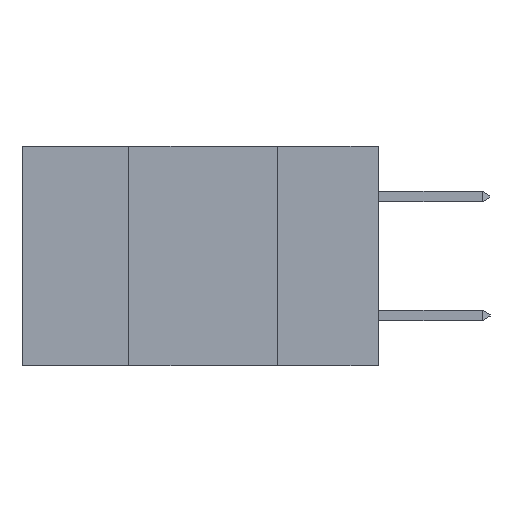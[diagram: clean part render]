
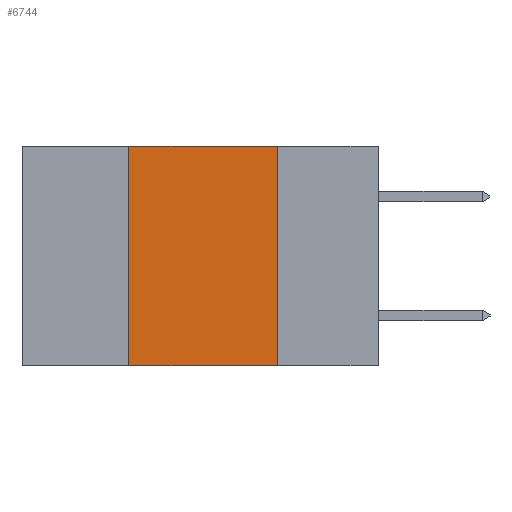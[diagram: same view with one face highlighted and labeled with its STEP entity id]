
A CAD part, left-side view. The second image highlights one B-rep face of the part: STEP entity #6744.
In plain terms, the highlighted planar face has unit normal (-1, 0, 0).
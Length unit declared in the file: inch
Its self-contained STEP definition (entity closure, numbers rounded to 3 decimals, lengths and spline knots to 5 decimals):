
#1080 = EDGE_LOOP ( 'NONE', ( #16471, #5968, #16943, #7786 ) ) ;
#1259 = VERTEX_POINT ( 'NONE', #9076 ) ;
#2033 = VECTOR ( 'NONE', #11052, 39.37008 ) ;
#2097 = VERTEX_POINT ( 'NONE', #18645 ) ;
#4067 = VERTEX_POINT ( 'NONE', #17515 ) ;
#4369 = CARTESIAN_POINT ( 'NONE',  ( 0., 0.6, -0.37 ) ) ;
#4642 = PLANE ( 'NONE',  #17692 ) ;
#4816 = CARTESIAN_POINT ( 'NONE',  ( 0., 0.42, 0. ) ) ;
#5235 = VECTOR ( 'NONE', #6069, 39.37008 ) ;
#5297 = FACE_OUTER_BOUND ( 'NONE', #1080, .T. ) ;
#5775 = LINE ( 'NONE', #4369, #5235 ) ;
#5968 = ORIENTED_EDGE ( 'NONE', *, *, #6484, .F. ) ;
#6069 = DIRECTION ( 'NONE',  ( 0., -1., 0. ) ) ;
#6484 = EDGE_CURVE ( 'NONE', #22376, #2097, #22396, .T. ) ;
#6744 = ADVANCED_FACE ( 'NONE', ( #5297 ), #4642, .F. ) ;
#7272 = CARTESIAN_POINT ( 'NONE',  ( 0., 0.42, -0.37 ) ) ;
#7786 = ORIENTED_EDGE ( 'NONE', *, *, #8800, .T. ) ;
#8374 = EDGE_CURVE ( 'NONE', #1259, #22376, #18796, .T. ) ;
#8800 = EDGE_CURVE ( 'NONE', #1259, #4067, #5775, .T. ) ;
#9076 = CARTESIAN_POINT ( 'NONE',  ( 0., 0.42, -0.37 ) ) ;
#9968 = DIRECTION ( 'NONE',  ( 1., 0., 0. ) ) ;
#10836 = DIRECTION ( 'NONE',  ( 0., 0., 1. ) ) ;
#11052 = DIRECTION ( 'NONE',  ( 0., -1., 0. ) ) ;
#12352 = LINE ( 'NONE', #13141, #21150 ) ;
#13141 = CARTESIAN_POINT ( 'NONE',  ( 0., 0.17, -0.37 ) ) ;
#13564 = EDGE_CURVE ( 'NONE', #2097, #4067, #12352, .T. ) ;
#14099 = VECTOR ( 'NONE', #10836, 39.37008 ) ;
#14932 = DIRECTION ( 'NONE',  ( 0., 0., -1. ) ) ;
#16471 = ORIENTED_EDGE ( 'NONE', *, *, #13564, .F. ) ;
#16943 = ORIENTED_EDGE ( 'NONE', *, *, #8374, .F. ) ;
#17515 = CARTESIAN_POINT ( 'NONE',  ( 0., 0.17, -0.37 ) ) ;
#17692 = AXIS2_PLACEMENT_3D ( 'NONE', #20530, #9968, #22273 ) ;
#18645 = CARTESIAN_POINT ( 'NONE',  ( 0., 0.17, 0. ) ) ;
#18796 = LINE ( 'NONE', #7272, #14099 ) ;
#19836 = CARTESIAN_POINT ( 'NONE',  ( 0., 0.6, 0. ) ) ;
#20530 = CARTESIAN_POINT ( 'NONE',  ( 0., 0.6, 0. ) ) ;
#21150 = VECTOR ( 'NONE', #14932, 39.37008 ) ;
#22273 = DIRECTION ( 'NONE',  ( 0., 0., -1. ) ) ;
#22376 = VERTEX_POINT ( 'NONE', #4816 ) ;
#22396 = LINE ( 'NONE', #19836, #2033 ) ;
